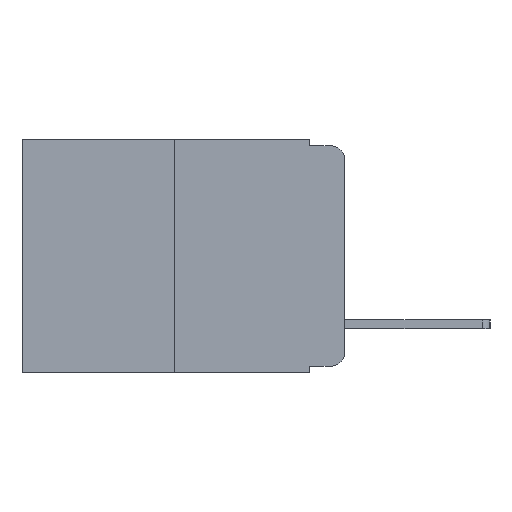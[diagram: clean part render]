
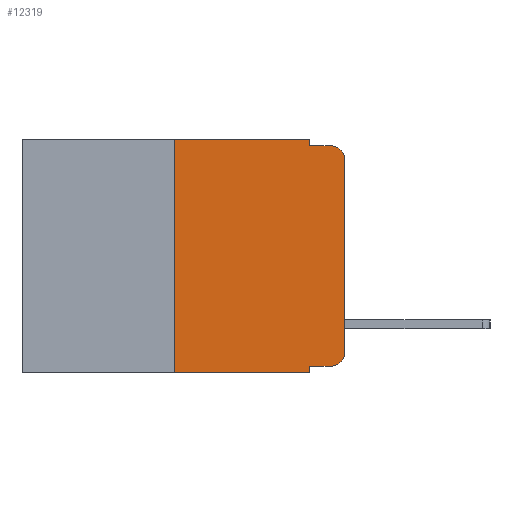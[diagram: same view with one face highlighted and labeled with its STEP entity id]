
A CAD part, left-side view. The second image highlights one B-rep face of the part: STEP entity #12319.
In plain terms, the highlighted planar face has unit normal (-1, 0, 0).
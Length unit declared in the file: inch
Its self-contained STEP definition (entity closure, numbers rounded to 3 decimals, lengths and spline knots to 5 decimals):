
#358 = VECTOR ( 'NONE', #12033, 39.37008 ) ;
#1454 = EDGE_CURVE ( 'NONE', #16910, #2215, #4017, .T. ) ;
#1568 = EDGE_CURVE ( 'NONE', #9442, #16848, #16477, .T. ) ;
#1593 = VECTOR ( 'NONE', #10544, 39.37008 ) ;
#1609 = CARTESIAN_POINT ( 'NONE',  ( 0., 0.25, -0.343 ) ) ;
#1615 = CARTESIAN_POINT ( 'NONE',  ( 0., 0.02, -0.03 ) ) ;
#1700 = ORIENTED_EDGE ( 'NONE', *, *, #12965, .T. ) ;
#1882 = CIRCLE ( 'NONE', #15555, 0.02 ) ;
#2215 = VERTEX_POINT ( 'NONE', #9362 ) ;
#2254 = CARTESIAN_POINT ( 'NONE',  ( 0., 0.051, -0.333 ) ) ;
#2434 = VERTEX_POINT ( 'NONE', #11736 ) ;
#2768 = ORIENTED_EDGE ( 'NONE', *, *, #6567, .T. ) ;
#2777 = LINE ( 'NONE', #16448, #5658 ) ;
#2899 = CARTESIAN_POINT ( 'NONE',  ( 0., 0.02, -0.333 ) ) ;
#2924 = CARTESIAN_POINT ( 'NONE',  ( 0., 0.473, 0. ) ) ;
#3027 = DIRECTION ( 'NONE',  ( 0., 0., -1. ) ) ;
#3310 = VERTEX_POINT ( 'NONE', #2899 ) ;
#3334 = FACE_OUTER_BOUND ( 'NONE', #7184, .T. ) ;
#3483 = DIRECTION ( 'NONE',  ( 0., -1., 0. ) ) ;
#3838 = ORIENTED_EDGE ( 'NONE', *, *, #11990, .T. ) ;
#3843 = VERTEX_POINT ( 'NONE', #8766 ) ;
#3886 = ORIENTED_EDGE ( 'NONE', *, *, #15690, .F. ) ;
#4017 = LINE ( 'NONE', #16316, #7360 ) ;
#4096 = LINE ( 'NONE', #14675, #358 ) ;
#4505 = VERTEX_POINT ( 'NONE', #1609 ) ;
#4567 = ORIENTED_EDGE ( 'NONE', *, *, #8672, .F. ) ;
#4569 = DIRECTION ( 'NONE',  ( 0., -1., 0. ) ) ;
#4582 = AXIS2_PLACEMENT_3D ( 'NONE', #1615, #11350, #3027 ) ;
#4740 = CARTESIAN_POINT ( 'NONE',  ( 0., 0., 0. ) ) ;
#5296 = CIRCLE ( 'NONE', #4582, 0.02 ) ;
#5658 = VECTOR ( 'NONE', #6939, 39.37008 ) ;
#5796 = VERTEX_POINT ( 'NONE', #2254 ) ;
#6567 = EDGE_CURVE ( 'NONE', #3310, #9442, #1882, .T. ) ;
#6939 = DIRECTION ( 'NONE',  ( 0., 0., 1. ) ) ;
#7180 = PLANE ( 'NONE',  #7192 ) ;
#7184 = EDGE_LOOP ( 'NONE', ( #13798, #1700, #3886, #16565, #4567, #9614, #3838, #9152, #11259, #2768 ) ) ;
#7192 = AXIS2_PLACEMENT_3D ( 'NONE', #2924, #16667, #8592 ) ;
#7360 = VECTOR ( 'NONE', #16684, 39.37008 ) ;
#7477 = VERTEX_POINT ( 'NONE', #9959 ) ;
#7656 = VECTOR ( 'NONE', #3483, 39.37008 ) ;
#8564 = VECTOR ( 'NONE', #17020, 39.37008 ) ;
#8592 = DIRECTION ( 'NONE',  ( 0., 0., -1. ) ) ;
#8672 = EDGE_CURVE ( 'NONE', #7477, #16910, #14441, .T. ) ;
#8766 = CARTESIAN_POINT ( 'NONE',  ( 0., 0.02, -0.01 ) ) ;
#8891 = CARTESIAN_POINT ( 'NONE',  ( 0., 0.051, -0.01 ) ) ;
#8999 = LINE ( 'NONE', #8891, #8564 ) ;
#9006 = EDGE_CURVE ( 'NONE', #4505, #7477, #2777, .T. ) ;
#9152 = ORIENTED_EDGE ( 'NONE', *, *, #16369, .F. ) ;
#9312 = VECTOR ( 'NONE', #15195, 39.37008 ) ;
#9362 = CARTESIAN_POINT ( 'NONE',  ( 0., 0.051, -0.01 ) ) ;
#9442 = VERTEX_POINT ( 'NONE', #14752 ) ;
#9614 = ORIENTED_EDGE ( 'NONE', *, *, #9006, .F. ) ;
#9943 = DIRECTION ( 'NONE',  ( 0., 0., -1. ) ) ;
#9959 = CARTESIAN_POINT ( 'NONE',  ( 0., 0.25, 0. ) ) ;
#9977 = DIRECTION ( 'NONE',  ( -1., 0., 0. ) ) ;
#10186 = CARTESIAN_POINT ( 'NONE',  ( 0., 0.02, -0.313 ) ) ;
#10544 = DIRECTION ( 'NONE',  ( 0., -1., 0. ) ) ;
#11259 = ORIENTED_EDGE ( 'NONE', *, *, #12419, .T. ) ;
#11350 = DIRECTION ( 'NONE',  ( -1., 0., 0. ) ) ;
#11736 = CARTESIAN_POINT ( 'NONE',  ( 0., 0.051, -0.343 ) ) ;
#11825 = CARTESIAN_POINT ( 'NONE',  ( 0., 0.473, 0. ) ) ;
#11990 = EDGE_CURVE ( 'NONE', #4505, #2434, #12678, .T. ) ;
#12033 = DIRECTION ( 'NONE',  ( 0., 0., -1. ) ) ;
#12239 = VECTOR ( 'NONE', #4569, 39.37008 ) ;
#12319 = ADVANCED_FACE ( 'NONE', ( #3334 ), #7180, .F. ) ;
#12419 = EDGE_CURVE ( 'NONE', #5796, #3310, #12658, .T. ) ;
#12576 = CARTESIAN_POINT ( 'NONE',  ( 0., 0.051, 0. ) ) ;
#12658 = LINE ( 'NONE', #16838, #12239 ) ;
#12678 = LINE ( 'NONE', #17256, #1593 ) ;
#12965 = EDGE_CURVE ( 'NONE', #16848, #3843, #5296, .T. ) ;
#13798 = ORIENTED_EDGE ( 'NONE', *, *, #1568, .T. ) ;
#14441 = LINE ( 'NONE', #11825, #7656 ) ;
#14675 = CARTESIAN_POINT ( 'NONE',  ( 0., 0.051, 0. ) ) ;
#14752 = CARTESIAN_POINT ( 'NONE',  ( 0., 0., -0.313 ) ) ;
#15195 = DIRECTION ( 'NONE',  ( 0., 0., 1. ) ) ;
#15555 = AXIS2_PLACEMENT_3D ( 'NONE', #10186, #9977, #9943 ) ;
#15690 = EDGE_CURVE ( 'NONE', #2215, #3843, #8999, .T. ) ;
#16316 = CARTESIAN_POINT ( 'NONE',  ( 0., 0.051, 0. ) ) ;
#16369 = EDGE_CURVE ( 'NONE', #5796, #2434, #4096, .T. ) ;
#16448 = CARTESIAN_POINT ( 'NONE',  ( 0., 0.25, 0. ) ) ;
#16477 = LINE ( 'NONE', #4740, #9312 ) ;
#16565 = ORIENTED_EDGE ( 'NONE', *, *, #1454, .F. ) ;
#16667 = DIRECTION ( 'NONE',  ( 1., 0., 0. ) ) ;
#16684 = DIRECTION ( 'NONE',  ( 0., 0., -1. ) ) ;
#16838 = CARTESIAN_POINT ( 'NONE',  ( 0., 0.051, -0.333 ) ) ;
#16848 = VERTEX_POINT ( 'NONE', #17592 ) ;
#16910 = VERTEX_POINT ( 'NONE', #12576 ) ;
#17020 = DIRECTION ( 'NONE',  ( 0., -1., 0. ) ) ;
#17256 = CARTESIAN_POINT ( 'NONE',  ( 0., 0.473, -0.343 ) ) ;
#17592 = CARTESIAN_POINT ( 'NONE',  ( 0., 0., -0.03 ) ) ;
